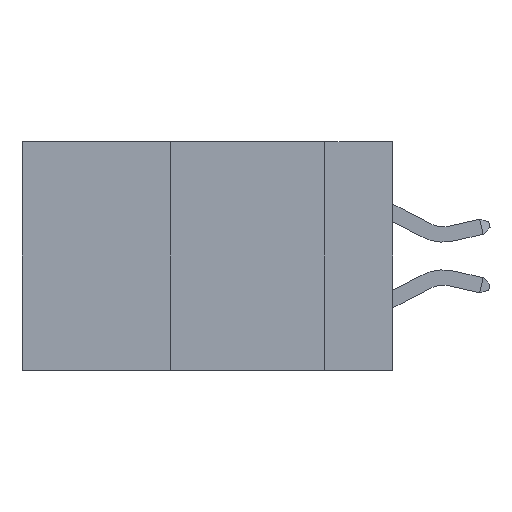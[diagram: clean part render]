
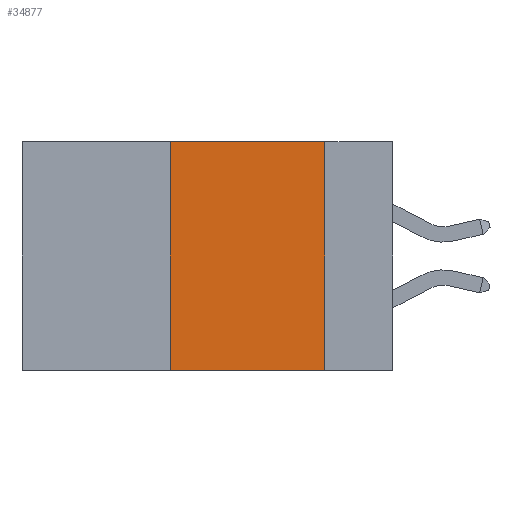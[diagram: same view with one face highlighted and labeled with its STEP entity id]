
A CAD part, left-side view. The second image highlights one B-rep face of the part: STEP entity #34877.
In plain terms, the highlighted planar face has unit normal (-1, 0, 0).
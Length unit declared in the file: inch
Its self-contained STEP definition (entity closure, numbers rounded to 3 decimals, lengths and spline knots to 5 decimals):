
#127 = LINE ( 'NONE', #33240, #16980 ) ;
#174 = CARTESIAN_POINT ( 'NONE',  ( 0., 0.6, 0. ) ) ;
#222 = LINE ( 'NONE', #27435, #30707 ) ;
#1161 = CARTESIAN_POINT ( 'NONE',  ( 0., 0.11, 0. ) ) ;
#4359 = FACE_OUTER_BOUND ( 'NONE', #24182, .T. ) ;
#5845 = DIRECTION ( 'NONE',  ( 0., -1., 0. ) ) ;
#6265 = ORIENTED_EDGE ( 'NONE', *, *, #27470, .F. ) ;
#6471 = EDGE_CURVE ( 'NONE', #23088, #38140, #222, .T. ) ;
#11025 = CARTESIAN_POINT ( 'NONE',  ( 0., 0.36, 0. ) ) ;
#11283 = ORIENTED_EDGE ( 'NONE', *, *, #6471, .F. ) ;
#11501 = DIRECTION ( 'NONE',  ( 0., 0., -1. ) ) ;
#14027 = DIRECTION ( 'NONE',  ( 0., 0., -1. ) ) ;
#16980 = VECTOR ( 'NONE', #5845, 39.37008 ) ;
#18223 = AXIS2_PLACEMENT_3D ( 'NONE', #31972, #25681, #14027 ) ;
#19485 = ORIENTED_EDGE ( 'NONE', *, *, #35456, .T. ) ;
#21970 = VERTEX_POINT ( 'NONE', #27726 ) ;
#22922 = PLANE ( 'NONE',  #18223 ) ;
#23088 = VERTEX_POINT ( 'NONE', #34657 ) ;
#24182 = EDGE_LOOP ( 'NONE', ( #27515, #6265, #11283, #19485 ) ) ;
#24422 = DIRECTION ( 'NONE',  ( 0., -1., 0. ) ) ;
#25681 = DIRECTION ( 'NONE',  ( 1., 0., 0. ) ) ;
#27435 = CARTESIAN_POINT ( 'NONE',  ( 0., 0.36, 0. ) ) ;
#27470 = EDGE_CURVE ( 'NONE', #38140, #35324, #33286, .T. ) ;
#27515 = ORIENTED_EDGE ( 'NONE', *, *, #28272, .F. ) ;
#27726 = CARTESIAN_POINT ( 'NONE',  ( 0., 0.11, -0.37 ) ) ;
#27995 = VECTOR ( 'NONE', #11501, 39.37008 ) ;
#28272 = EDGE_CURVE ( 'NONE', #35324, #21970, #32820, .T. ) ;
#30707 = VECTOR ( 'NONE', #33330, 39.37008 ) ;
#31972 = CARTESIAN_POINT ( 'NONE',  ( 0., 0.6, 0. ) ) ;
#32335 = VECTOR ( 'NONE', #24422, 39.37008 ) ;
#32610 = CARTESIAN_POINT ( 'NONE',  ( 0., 0.11, 0. ) ) ;
#32820 = LINE ( 'NONE', #32610, #27995 ) ;
#33240 = CARTESIAN_POINT ( 'NONE',  ( 0., 0.6, -0.37 ) ) ;
#33286 = LINE ( 'NONE', #174, #32335 ) ;
#33330 = DIRECTION ( 'NONE',  ( 0., 0., 1. ) ) ;
#34657 = CARTESIAN_POINT ( 'NONE',  ( 0., 0.36, -0.37 ) ) ;
#34877 = ADVANCED_FACE ( 'NONE', ( #4359 ), #22922, .F. ) ;
#35324 = VERTEX_POINT ( 'NONE', #1161 ) ;
#35456 = EDGE_CURVE ( 'NONE', #23088, #21970, #127, .T. ) ;
#38140 = VERTEX_POINT ( 'NONE', #11025 ) ;
